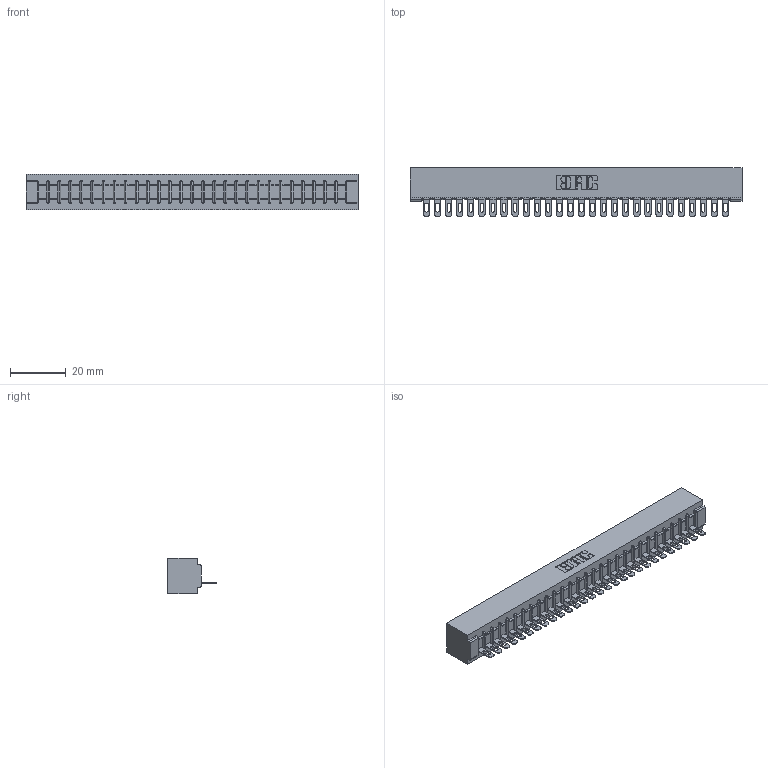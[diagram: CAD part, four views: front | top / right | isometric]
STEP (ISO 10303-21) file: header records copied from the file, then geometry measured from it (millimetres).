
FILE_DESCRIPTION (( 'STEP AP203' ), '1' );
FILE_NAME ('357-028-501-101.STEP', '2018-08-09T05:53:09', ( '' ), ( '' ), 'SwSTEP 2.0', 'SolidWorks 2016', '' );
FILE_SCHEMA (( 'CONFIG_CONTROL_DESIGN' ));
Length unit declared in the file: inch
Products named in the file (3): 307 Part_No Mounting Lugs; 307-290-002_501; 357-028-501-101
Assembly tree (29 placements, depth 2):
  357-028-501-101
    307 Part_No Mounting Lugs
    307-290-002_501  x28
Bounding box: 118.82 x 17.42 x 12.7 mm (x, y, z)
Volume: 13193.1 mm3; surface area: 16820.8 mm2
Topology: 29 solids, 29 shells, 2267 faces, 6963 edges, 4562 vertices
Faces by surface type: plane 1298, cylinder 911, sphere 58
Entity records: 26246 total; most frequent: CARTESIAN_POINT 4424, ORIENTED_EDGE 4414, DIRECTION 4307, EDGE_CURVE 2207, VECTOR 1681, LINE 1681, VERTEX_POINT 1430, AXIS2_PLACEMENT_3D 1313
